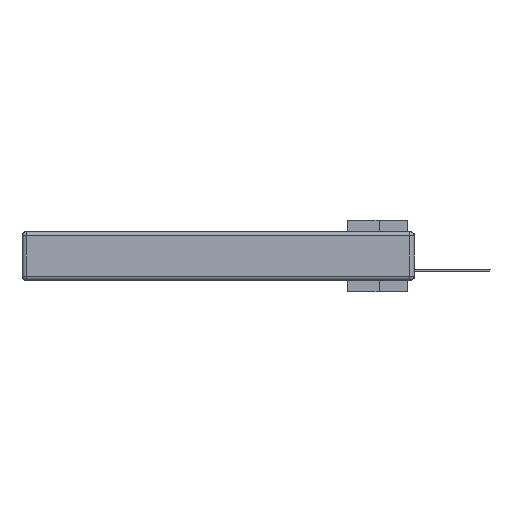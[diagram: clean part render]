
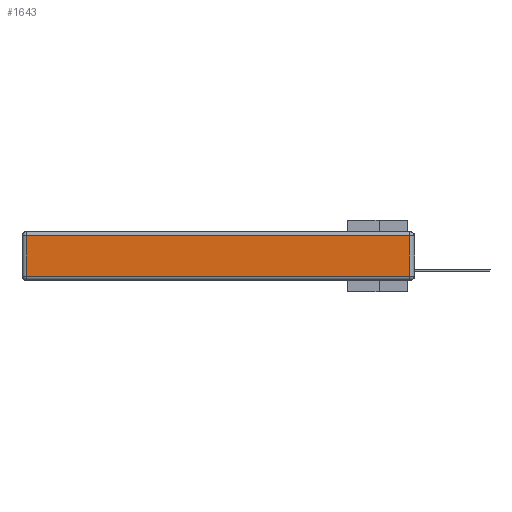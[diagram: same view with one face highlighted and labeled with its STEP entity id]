
A CAD part, left-side view. The second image highlights one B-rep face of the part: STEP entity #1643.
In plain terms, the highlighted planar face has unit normal (-1, 0, 0).
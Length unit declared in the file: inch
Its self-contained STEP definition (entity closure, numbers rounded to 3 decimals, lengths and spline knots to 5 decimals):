
#1251 = CARTESIAN_POINT ( 'NONE',  ( 0., 2.75, -0.03 ) ) ;
#1643 = ADVANCED_FACE ( 'NONE', ( #28256 ), #20137, .T. ) ;
#1657 = VERTEX_POINT ( 'NONE', #25087 ) ;
#2673 = LINE ( 'NONE', #6499, #9735 ) ;
#2741 = VECTOR ( 'NONE', #14354, 39.37008 ) ;
#3612 = CARTESIAN_POINT ( 'NONE',  ( 0., 2.72, -0.03 ) ) ;
#4512 = EDGE_CURVE ( 'NONE', #1657, #10402, #11441, .T. ) ;
#4949 = VERTEX_POINT ( 'NONE', #9627 ) ;
#6499 = CARTESIAN_POINT ( 'NONE',  ( 0., 2.72, -0.343 ) ) ;
#8595 = EDGE_CURVE ( 'NONE', #10402, #9349, #2673, .T. ) ;
#9349 = VERTEX_POINT ( 'NONE', #25685 ) ;
#9400 = AXIS2_PLACEMENT_3D ( 'NONE', #33754, #33644, #17495 ) ;
#9627 = CARTESIAN_POINT ( 'NONE',  ( 0., 0.03, -0.313 ) ) ;
#9735 = VECTOR ( 'NONE', #27791, 39.37008 ) ;
#9737 = LINE ( 'NONE', #12554, #25056 ) ;
#10192 = ORIENTED_EDGE ( 'NONE', *, *, #8595, .T. ) ;
#10402 = VERTEX_POINT ( 'NONE', #3612 ) ;
#11441 = LINE ( 'NONE', #1251, #2741 ) ;
#12164 = CARTESIAN_POINT ( 'NONE',  ( 0., 0., -0.313 ) ) ;
#12554 = CARTESIAN_POINT ( 'NONE',  ( 0., 0.03, -0.343 ) ) ;
#14354 = DIRECTION ( 'NONE',  ( 0., 1., 0. ) ) ;
#17495 = DIRECTION ( 'NONE',  ( 0., 0., 1. ) ) ;
#17961 = DIRECTION ( 'NONE',  ( 0., 0., 1. ) ) ;
#19543 = EDGE_CURVE ( 'NONE', #9349, #4949, #24179, .T. ) ;
#20137 = PLANE ( 'NONE',  #9400 ) ;
#20970 = ORIENTED_EDGE ( 'NONE', *, *, #4512, .T. ) ;
#22538 = DIRECTION ( 'NONE',  ( 0., -1., 0. ) ) ;
#24179 = LINE ( 'NONE', #12164, #30434 ) ;
#25056 = VECTOR ( 'NONE', #17961, 39.37008 ) ;
#25087 = CARTESIAN_POINT ( 'NONE',  ( 0., 0.03, -0.03 ) ) ;
#25383 = ORIENTED_EDGE ( 'NONE', *, *, #19543, .T. ) ;
#25543 = EDGE_CURVE ( 'NONE', #4949, #1657, #9737, .T. ) ;
#25685 = CARTESIAN_POINT ( 'NONE',  ( 0., 2.72, -0.313 ) ) ;
#27791 = DIRECTION ( 'NONE',  ( 0., 0., -1. ) ) ;
#28256 = FACE_OUTER_BOUND ( 'NONE', #34263, .T. ) ;
#30434 = VECTOR ( 'NONE', #22538, 39.37008 ) ;
#33644 = DIRECTION ( 'NONE',  ( -1., 0., 0. ) ) ;
#33754 = CARTESIAN_POINT ( 'NONE',  ( 0., 0., -0.343 ) ) ;
#34125 = ORIENTED_EDGE ( 'NONE', *, *, #25543, .T. ) ;
#34263 = EDGE_LOOP ( 'NONE', ( #25383, #34125, #20970, #10192 ) ) ;
